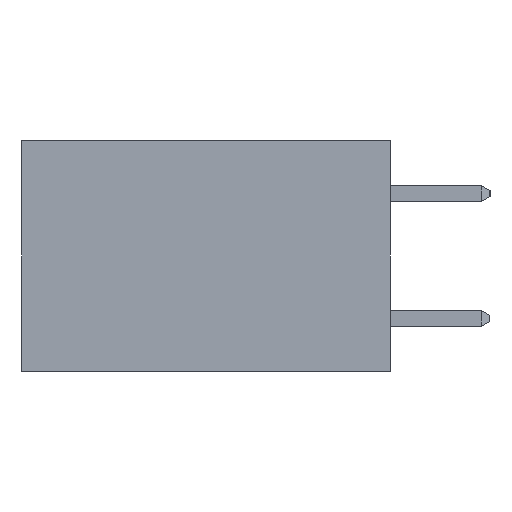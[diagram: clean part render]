
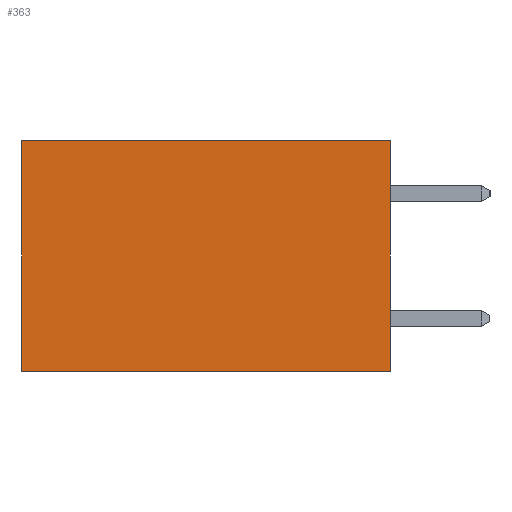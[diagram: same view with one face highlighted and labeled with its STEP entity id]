
A CAD part, left-side view. The second image highlights one B-rep face of the part: STEP entity #363.
In plain terms, the highlighted planar face has unit normal (-1, 0, 0).
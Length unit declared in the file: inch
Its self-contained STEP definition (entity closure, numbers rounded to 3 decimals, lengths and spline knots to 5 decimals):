
#198 = VECTOR ( 'NONE', #4783, 39.37008 ) ;
#271 = CARTESIAN_POINT ( 'NONE',  ( 0.277, 0.59, -0.37 ) ) ;
#363 = ADVANCED_FACE ( 'NONE', ( #2432 ), #788, .F. ) ;
#754 = VECTOR ( 'NONE', #7330, 39.37008 ) ;
#788 = PLANE ( 'NONE',  #6868 ) ;
#853 = CARTESIAN_POINT ( 'NONE',  ( 0.277, 0., -0.37 ) ) ;
#1820 = DIRECTION ( 'NONE',  ( 1., 0., 0. ) ) ;
#1966 = DIRECTION ( 'NONE',  ( 0., 0., -1. ) ) ;
#2129 = CARTESIAN_POINT ( 'NONE',  ( 0.277, 0., 0. ) ) ;
#2432 = FACE_OUTER_BOUND ( 'NONE', #7875, .T. ) ;
#2482 = VERTEX_POINT ( 'NONE', #10414 ) ;
#2955 = EDGE_CURVE ( 'NONE', #10849, #7781, #8123, .T. ) ;
#3456 = LINE ( 'NONE', #2129, #754 ) ;
#4109 = ORIENTED_EDGE ( 'NONE', *, *, #9625, .T. ) ;
#4682 = DIRECTION ( 'NONE',  ( 0., 0., -1. ) ) ;
#4718 = CARTESIAN_POINT ( 'NONE',  ( 0.277, 0., -0.37 ) ) ;
#4783 = DIRECTION ( 'NONE',  ( 0., 1., 0. ) ) ;
#5443 = ORIENTED_EDGE ( 'NONE', *, *, #2955, .F. ) ;
#6088 = EDGE_CURVE ( 'NONE', #9329, #7781, #10586, .T. ) ;
#6868 = AXIS2_PLACEMENT_3D ( 'NONE', #8815, #1820, #1966 ) ;
#7326 = EDGE_CURVE ( 'NONE', #2482, #10849, #13085, .T. ) ;
#7330 = DIRECTION ( 'NONE',  ( 0., 1., 0. ) ) ;
#7352 = ORIENTED_EDGE ( 'NONE', *, *, #6088, .T. ) ;
#7506 = CARTESIAN_POINT ( 'NONE',  ( 0.277, 0.59, -0.37 ) ) ;
#7691 = DIRECTION ( 'NONE',  ( 0., 0., -1. ) ) ;
#7781 = VERTEX_POINT ( 'NONE', #271 ) ;
#7875 = EDGE_LOOP ( 'NONE', ( #7352, #5443, #13174, #4109 ) ) ;
#8123 = LINE ( 'NONE', #8332, #198 ) ;
#8168 = VECTOR ( 'NONE', #7691, 39.37008 ) ;
#8332 = CARTESIAN_POINT ( 'NONE',  ( 0.277, 0., -0.37 ) ) ;
#8815 = CARTESIAN_POINT ( 'NONE',  ( 0.277, 0., -0.37 ) ) ;
#9329 = VERTEX_POINT ( 'NONE', #12977 ) ;
#9625 = EDGE_CURVE ( 'NONE', #2482, #9329, #3456, .T. ) ;
#10414 = CARTESIAN_POINT ( 'NONE',  ( 0.277, 0., 0. ) ) ;
#10586 = LINE ( 'NONE', #7506, #8168 ) ;
#10849 = VERTEX_POINT ( 'NONE', #853 ) ;
#12768 = VECTOR ( 'NONE', #4682, 39.37008 ) ;
#12977 = CARTESIAN_POINT ( 'NONE',  ( 0.277, 0.59, 0. ) ) ;
#13085 = LINE ( 'NONE', #4718, #12768 ) ;
#13174 = ORIENTED_EDGE ( 'NONE', *, *, #7326, .F. ) ;
